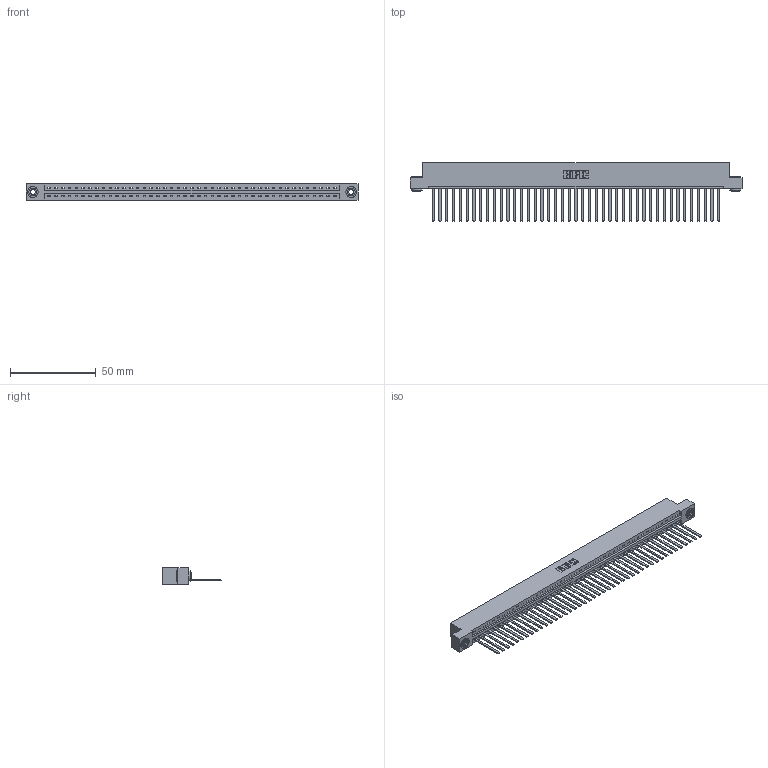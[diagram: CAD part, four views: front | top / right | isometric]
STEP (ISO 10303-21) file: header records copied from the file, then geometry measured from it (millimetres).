
FILE_DESCRIPTION (( 'STEP AP203' ), '1' );
FILE_NAME ('387-043-544-103.STEP', '2019-10-04T22:38:02', ( '' ), ( '' ), 'SwSTEP 2.0', 'SolidWorks 2016', '' );
FILE_SCHEMA (( 'CONFIG_CONTROL_DESIGN' ));
Length unit declared in the file: inch
Products named in the file (4): 345-292-001_345-293-144; 345-250-002_345-250-002-102; 337 Part_Flush Mounting Lugs - 0.156 Dia-TH; 387-043-544-103
Assembly tree (46 placements, depth 2):
  387-043-544-103
    337 Part_Flush Mounting Lugs - 0.156 Dia-TH
    345-292-001_345-293-144  x43
    345-250-002_345-250-002-102  x2
Bounding box: 193.4 x 34.3 x 9.4 mm (x, y, z)
Volume: 20630.1 mm3; surface area: 23194.6 mm2
Topology: 46 solids, 46 shells, 2560 faces, 7697 edges, 5070 vertices
Faces by surface type: plane 1886, cylinder 666, cone 8
Entity records: 32300 total; most frequent: CARTESIAN_POINT 5602, ORIENTED_EDGE 5574, DIRECTION 4743, EDGE_CURVE 2787, LINE 2639, VECTOR 2639, VERTEX_POINT 1854, AXIS2_PLACEMENT_3D 1052
